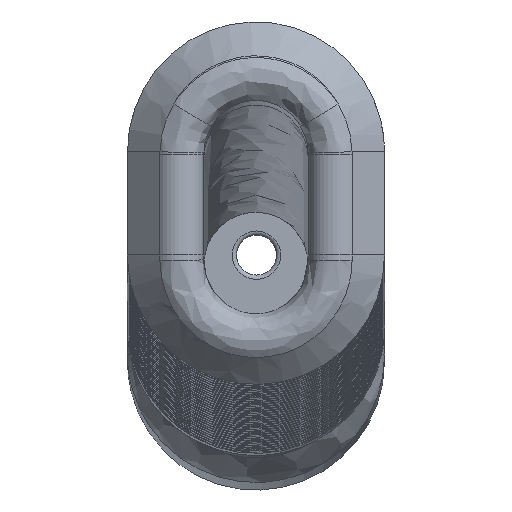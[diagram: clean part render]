
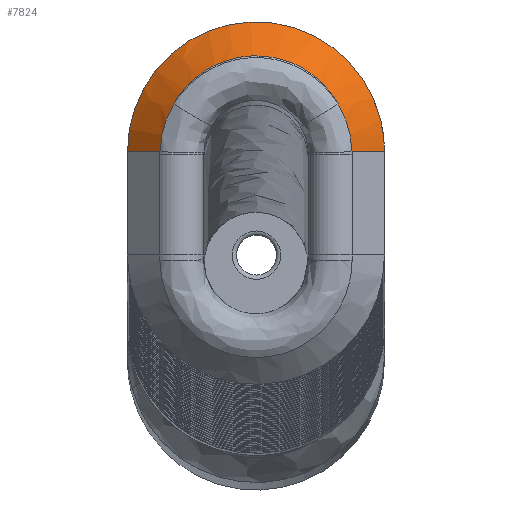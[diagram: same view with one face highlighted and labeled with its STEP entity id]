
A CAD part, front view. The second image highlights one B-rep face of the part: STEP entity #7824.
In plain terms, the highlighted free-form (B-spline) face has degree [3, 3] with [4, 10] control points.
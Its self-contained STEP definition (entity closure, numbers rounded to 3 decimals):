
#497=LINE('',#13950,#845);
#500=LINE('',#14000,#848);
#845=VECTOR('',#9330,10.);
#848=VECTOR('',#9333,10.);
#1272=ELLIPSE('',#8436,15.113,15.);
#1348=FACE_OUTER_BOUND('',#1926,.T.);
#1926=EDGE_LOOP('',(#5686,#5687,#5688,#5689,#5690,#5691));
#2466=B_SPLINE_CURVE_WITH_KNOTS('',3,(#13674,#13675,#13676,#13677),
 .UNSPECIFIED.,.F.,.F.,(4,4),(-0.474,0.),.UNSPECIFIED.);
#2468=B_SPLINE_CURVE_WITH_KNOTS('',3,(#13743,#13744,#13745,#13746),
 .UNSPECIFIED.,.F.,.F.,(4,4),(-0.474,0.),.UNSPECIFIED.);
#2475=B_SPLINE_CURVE_WITH_KNOTS('',3,(#13993,#13994,#13995,#13996,#13997,
#13998,#13999),.UNSPECIFIED.,.F.,.F.,(4,1,1,1,4),(-1.61,-1.243,
-0.875,-0.691,-0.324),.UNSPECIFIED.);
#3291=VERTEX_POINT('',#11250);
#3292=VERTEX_POINT('',#11252);
#3439=VERTEX_POINT('',#13634);
#3440=VERTEX_POINT('',#13636);
#3441=VERTEX_POINT('',#13673);
#3443=VERTEX_POINT('',#13741);
#4123=EDGE_CURVE('',#3291,#3292,#1272,.T.);
#4282=EDGE_CURVE('',#3440,#3441,#2466,.T.);
#4287=EDGE_CURVE('',#3443,#3439,#2468,.T.);
#4303=EDGE_CURVE('',#3291,#3441,#497,.T.);
#4306=EDGE_CURVE('',#3439,#3440,#2475,.T.);
#4307=EDGE_CURVE('',#3292,#3443,#500,.T.);
#5686=ORIENTED_EDGE('',*,*,#4282,.F.);
#5687=ORIENTED_EDGE('',*,*,#4306,.F.);
#5688=ORIENTED_EDGE('',*,*,#4287,.F.);
#5689=ORIENTED_EDGE('',*,*,#4307,.F.);
#5690=ORIENTED_EDGE('',*,*,#4123,.F.);
#5691=ORIENTED_EDGE('',*,*,#4303,.T.);
#7588=B_SPLINE_SURFACE_WITH_KNOTS('',3,3,((#13953,#13954,#13955,#13956,
#13957,#13958,#13959,#13960,#13961,#13962),(#13963,#13964,#13965,#13966,
#13967,#13968,#13969,#13970,#13971,#13972),(#13973,#13974,#13975,#13976,
#13977,#13978,#13979,#13980,#13981,#13982),(#13983,#13984,#13985,#13986,
#13987,#13988,#13989,#13990,#13991,#13992)),.UNSPECIFIED.,.F.,.F.,.F.,(4,
4),(4,1,1,1,1,1,1,4),(0.342,1.),(-1.571,-1.122,
-0.673,-0.224,0.224,0.673,
1.122,1.571),.UNSPECIFIED.);
#7824=ADVANCED_FACE('',(#1348),#7588,.T.);
#8436=AXIS2_PLACEMENT_3D('',#11253,#9215,#9216);
#9215=DIRECTION('center_axis',(0.,1.,0.));
#9216=DIRECTION('ref_axis',(0.,0.,1.));
#9330=DIRECTION('',(0.707,-0.707,0.));
#9333=DIRECTION('',(-0.707,-0.707,0.));
#11250=CARTESIAN_POINT('',(63.916,-101.,186.839));
#11252=CARTESIAN_POINT('',(93.916,-101.,186.839));
#11253=CARTESIAN_POINT('Origin',(78.916,-101.,186.839));
#13634=CARTESIAN_POINT('',(88.513,-104.95,192.372));
#13636=CARTESIAN_POINT('',(69.319,-104.95,192.372));
#13673=CARTESIAN_POINT('',(67.702,-104.786,186.839));
#13674=CARTESIAN_POINT('Ctrl Pts',(69.319,-104.95,192.372));
#13675=CARTESIAN_POINT('Ctrl Pts',(68.324,-104.907,190.698));
#13676=CARTESIAN_POINT('Ctrl Pts',(67.768,-104.852,188.774));
#13677=CARTESIAN_POINT('Ctrl Pts',(67.702,-104.786,186.839));
#13741=CARTESIAN_POINT('',(90.129,-104.786,186.839));
#13743=CARTESIAN_POINT('Ctrl Pts',(90.129,-104.786,186.839));
#13744=CARTESIAN_POINT('Ctrl Pts',(90.064,-104.852,188.774));
#13745=CARTESIAN_POINT('Ctrl Pts',(89.508,-104.907,190.698));
#13746=CARTESIAN_POINT('Ctrl Pts',(88.513,-104.95,192.372));
#13950=CARTESIAN_POINT('',(63.916,-101.,186.839));
#13953=CARTESIAN_POINT('Ctrl Pts',(89.966,-104.95,186.839));
#13954=CARTESIAN_POINT('Ctrl Pts',(89.966,-104.95,188.513));
#13955=CARTESIAN_POINT('Ctrl Pts',(89.207,-104.95,191.86));
#13956=CARTESIAN_POINT('Ctrl Pts',(86.028,-104.95,195.876));
#13957=CARTESIAN_POINT('Ctrl Pts',(81.451,-104.95,198.092));
#13958=CARTESIAN_POINT('Ctrl Pts',(76.381,-104.95,198.095));
#13959=CARTESIAN_POINT('Ctrl Pts',(71.805,-104.95,195.874));
#13960=CARTESIAN_POINT('Ctrl Pts',(68.624,-104.95,191.862));
#13961=CARTESIAN_POINT('Ctrl Pts',(67.865,-104.95,188.513));
#13962=CARTESIAN_POINT('Ctrl Pts',(67.865,-104.95,186.839));
#13963=CARTESIAN_POINT('Ctrl Pts',(91.283,-103.633,186.839));
#13964=CARTESIAN_POINT('Ctrl Pts',(91.283,-103.633,188.708));
#13965=CARTESIAN_POINT('Ctrl Pts',(90.435,-103.633,192.446));
#13966=CARTESIAN_POINT('Ctrl Pts',(86.882,-103.633,196.938));
#13967=CARTESIAN_POINT('Ctrl Pts',(81.756,-103.633,199.42));
#13968=CARTESIAN_POINT('Ctrl Pts',(76.075,-103.633,199.423));
#13969=CARTESIAN_POINT('Ctrl Pts',(70.952,-103.633,196.935));
#13970=CARTESIAN_POINT('Ctrl Pts',(67.395,-103.633,192.448));
#13971=CARTESIAN_POINT('Ctrl Pts',(66.549,-103.633,188.708));
#13972=CARTESIAN_POINT('Ctrl Pts',(66.549,-103.633,186.839));
#13973=CARTESIAN_POINT('Ctrl Pts',(92.599,-102.317,186.839));
#13974=CARTESIAN_POINT('Ctrl Pts',(92.599,-102.317,188.904));
#13975=CARTESIAN_POINT('Ctrl Pts',(91.663,-102.317,193.033));
#13976=CARTESIAN_POINT('Ctrl Pts',(87.735,-102.317,197.999));
#13977=CARTESIAN_POINT('Ctrl Pts',(82.062,-102.317,200.747));
#13978=CARTESIAN_POINT('Ctrl Pts',(75.769,-102.317,200.75));
#13979=CARTESIAN_POINT('Ctrl Pts',(70.098,-102.317,197.996));
#13980=CARTESIAN_POINT('Ctrl Pts',(66.167,-102.317,193.035));
#13981=CARTESIAN_POINT('Ctrl Pts',(65.232,-102.317,188.904));
#13982=CARTESIAN_POINT('Ctrl Pts',(65.232,-102.317,186.839));
#13983=CARTESIAN_POINT('Ctrl Pts',(93.916,-101.,186.839));
#13984=CARTESIAN_POINT('Ctrl Pts',(93.916,-101.,189.099));
#13985=CARTESIAN_POINT('Ctrl Pts',(92.891,-101.,193.619));
#13986=CARTESIAN_POINT('Ctrl Pts',(88.589,-101.,199.06));
#13987=CARTESIAN_POINT('Ctrl Pts',(82.367,-101.,202.074));
#13988=CARTESIAN_POINT('Ctrl Pts',(75.464,-101.,202.078));
#13989=CARTESIAN_POINT('Ctrl Pts',(69.245,-101.,199.057));
#13990=CARTESIAN_POINT('Ctrl Pts',(64.939,-101.,193.621));
#13991=CARTESIAN_POINT('Ctrl Pts',(63.916,-101.,189.099));
#13992=CARTESIAN_POINT('Ctrl Pts',(63.916,-101.,186.839));
#13993=CARTESIAN_POINT('Ctrl Pts',(88.513,-104.95,192.372));
#13994=CARTESIAN_POINT('Ctrl Pts',(87.432,-104.95,194.285));
#13995=CARTESIAN_POINT('Ctrl Pts',(84.089,-104.95,197.491));
#13996=CARTESIAN_POINT('Ctrl Pts',(78.296,-104.95,198.392));
#13997=CARTESIAN_POINT('Ctrl Pts',(72.906,-104.95,196.673));
#13998=CARTESIAN_POINT('Ctrl Pts',(70.399,-104.95,194.285));
#13999=CARTESIAN_POINT('Ctrl Pts',(69.319,-104.95,192.372));
#14000=CARTESIAN_POINT('',(93.916,-101.,186.839));
